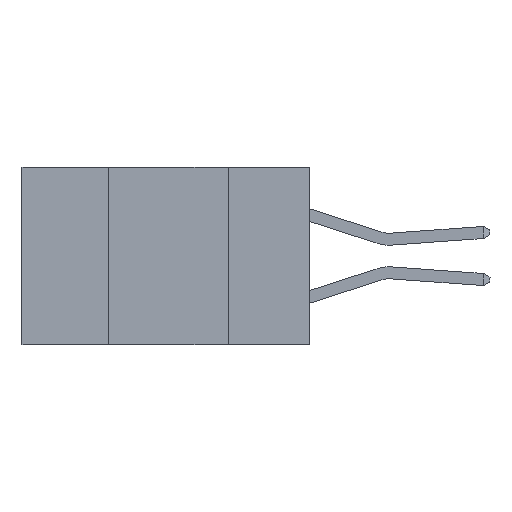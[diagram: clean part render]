
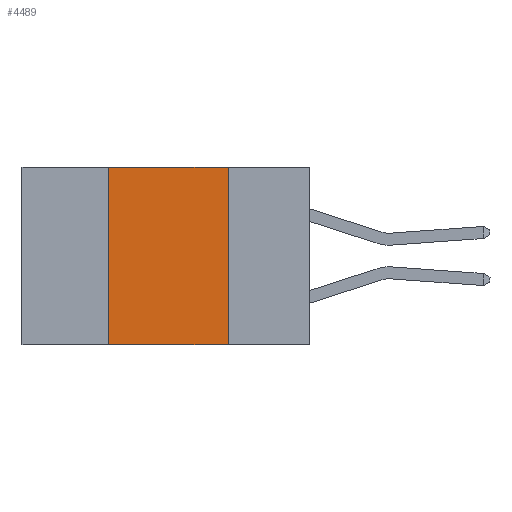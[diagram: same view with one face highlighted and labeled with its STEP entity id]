
A CAD part, left-side view. The second image highlights one B-rep face of the part: STEP entity #4489.
In plain terms, the highlighted planar face has unit normal (-1, 0, 0).
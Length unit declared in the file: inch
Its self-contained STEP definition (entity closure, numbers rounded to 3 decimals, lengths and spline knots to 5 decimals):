
#23 = VECTOR ( 'NONE', #7612, 39.37008 ) ;
#271 = VECTOR ( 'NONE', #5807, 39.37008 ) ;
#631 = LINE ( 'NONE', #1993, #17483 ) ;
#1379 = DIRECTION ( 'NONE',  ( 1., 0., 0. ) ) ;
#1993 = CARTESIAN_POINT ( 'NONE',  ( 0., 0.17, 0. ) ) ;
#2538 = VERTEX_POINT ( 'NONE', #13029 ) ;
#3215 = FACE_OUTER_BOUND ( 'NONE', #3637, .T. ) ;
#3325 = CARTESIAN_POINT ( 'NONE',  ( 0., 0.17, -0.37 ) ) ;
#3637 = EDGE_LOOP ( 'NONE', ( #5390, #20924, #9311, #13801 ) ) ;
#3639 = AXIS2_PLACEMENT_3D ( 'NONE', #11333, #1379, #13246 ) ;
#4489 = ADVANCED_FACE ( 'NONE', ( #3215 ), #21401, .F. ) ;
#4920 = LINE ( 'NONE', #6838, #14823 ) ;
#5390 = ORIENTED_EDGE ( 'NONE', *, *, #6673, .F. ) ;
#5807 = DIRECTION ( 'NONE',  ( 0., -1., 0. ) ) ;
#5968 = VERTEX_POINT ( 'NONE', #3325 ) ;
#6484 = CARTESIAN_POINT ( 'NONE',  ( 0., 0.42, -0.37 ) ) ;
#6673 = EDGE_CURVE ( 'NONE', #13602, #5968, #631, .T. ) ;
#6838 = CARTESIAN_POINT ( 'NONE',  ( 0., 0.6, -0.37 ) ) ;
#7612 = DIRECTION ( 'NONE',  ( 0., 0., 1. ) ) ;
#9311 = ORIENTED_EDGE ( 'NONE', *, *, #16702, .F. ) ;
#11333 = CARTESIAN_POINT ( 'NONE',  ( 0., 0.6, 0. ) ) ;
#11898 = DIRECTION ( 'NONE',  ( 0., -1., 0. ) ) ;
#12104 = VERTEX_POINT ( 'NONE', #6484 ) ;
#12561 = CARTESIAN_POINT ( 'NONE',  ( 0., 0.6, 0. ) ) ;
#13029 = CARTESIAN_POINT ( 'NONE',  ( 0., 0.42, 0. ) ) ;
#13246 = DIRECTION ( 'NONE',  ( 0., 0., -1. ) ) ;
#13593 = LINE ( 'NONE', #15915, #23 ) ;
#13602 = VERTEX_POINT ( 'NONE', #20042 ) ;
#13801 = ORIENTED_EDGE ( 'NONE', *, *, #14490, .T. ) ;
#14047 = EDGE_CURVE ( 'NONE', #2538, #13602, #21513, .T. ) ;
#14490 = EDGE_CURVE ( 'NONE', #12104, #5968, #4920, .T. ) ;
#14823 = VECTOR ( 'NONE', #11898, 39.37008 ) ;
#15453 = DIRECTION ( 'NONE',  ( 0., 0., -1. ) ) ;
#15915 = CARTESIAN_POINT ( 'NONE',  ( 0., 0.42, 0. ) ) ;
#16702 = EDGE_CURVE ( 'NONE', #12104, #2538, #13593, .T. ) ;
#17483 = VECTOR ( 'NONE', #15453, 39.37008 ) ;
#20042 = CARTESIAN_POINT ( 'NONE',  ( 0., 0.17, 0. ) ) ;
#20924 = ORIENTED_EDGE ( 'NONE', *, *, #14047, .F. ) ;
#21401 = PLANE ( 'NONE',  #3639 ) ;
#21513 = LINE ( 'NONE', #12561, #271 ) ;
